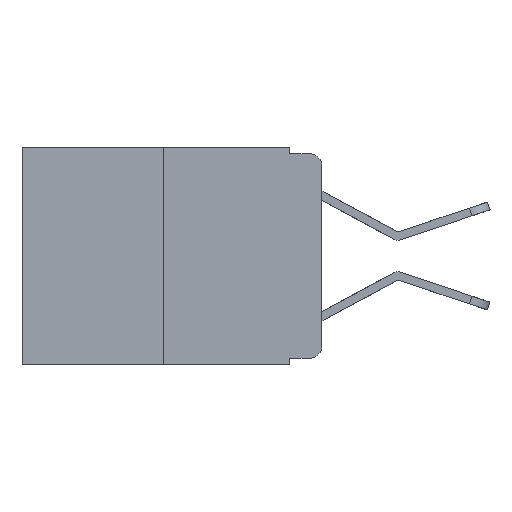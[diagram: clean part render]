
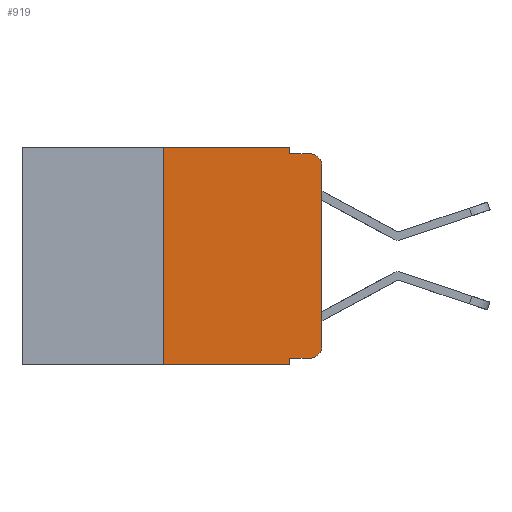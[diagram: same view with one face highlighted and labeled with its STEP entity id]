
A CAD part, left-side view. The second image highlights one B-rep face of the part: STEP entity #919.
In plain terms, the highlighted planar face has unit normal (-1, 0, 0).
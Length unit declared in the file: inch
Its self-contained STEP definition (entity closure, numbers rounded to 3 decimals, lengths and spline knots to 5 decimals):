
#36 = LINE ( 'NONE', #2235, #15586 ) ;
#129 = AXIS2_PLACEMENT_3D ( 'NONE', #6723, #17205, #8230 ) ;
#309 = LINE ( 'NONE', #2579, #7879 ) ;
#554 = ORIENTED_EDGE ( 'NONE', *, *, #718, .F. ) ;
#718 = EDGE_CURVE ( 'NONE', #16285, #2313, #2250, .T. ) ;
#919 = ADVANCED_FACE ( 'NONE', ( #9537 ), #12944, .F. ) ;
#1104 = DIRECTION ( 'NONE',  ( 1., 0., 0. ) ) ;
#1184 = EDGE_CURVE ( 'NONE', #2313, #10644, #309, .T. ) ;
#1621 = LINE ( 'NONE', #5008, #17148 ) ;
#2152 = EDGE_CURVE ( 'NONE', #19478, #2261, #36, .T. ) ;
#2235 = CARTESIAN_POINT ( 'NONE',  ( 0., 0.051, 0. ) ) ;
#2250 = LINE ( 'NONE', #16620, #9306 ) ;
#2261 = VERTEX_POINT ( 'NONE', #2502 ) ;
#2296 = DIRECTION ( 'NONE',  ( 0., 0., -1. ) ) ;
#2313 = VERTEX_POINT ( 'NONE', #13131 ) ;
#2376 = CARTESIAN_POINT ( 'NONE',  ( 0., 0.473, -0.343 ) ) ;
#2391 = EDGE_CURVE ( 'NONE', #10644, #11208, #12288, .T. ) ;
#2502 = CARTESIAN_POINT ( 'NONE',  ( 0., 0.051, -0.343 ) ) ;
#2579 = CARTESIAN_POINT ( 'NONE',  ( 0., 0.473, 0. ) ) ;
#2669 = DIRECTION ( 'NONE',  ( -1., 0., 0. ) ) ;
#3202 = VERTEX_POINT ( 'NONE', #13690 ) ;
#3598 = VECTOR ( 'NONE', #7620, 39.37008 ) ;
#3809 = VERTEX_POINT ( 'NONE', #4970 ) ;
#3857 = VECTOR ( 'NONE', #10298, 39.37008 ) ;
#3967 = CARTESIAN_POINT ( 'NONE',  ( 0., 0., -0.03 ) ) ;
#4226 = VERTEX_POINT ( 'NONE', #10428 ) ;
#4970 = CARTESIAN_POINT ( 'NONE',  ( 0., 0.02, -0.333 ) ) ;
#5008 = CARTESIAN_POINT ( 'NONE',  ( 0., 0., 0. ) ) ;
#5072 = ORIENTED_EDGE ( 'NONE', *, *, #16194, .F. ) ;
#5185 = EDGE_CURVE ( 'NONE', #4226, #17462, #1621, .T. ) ;
#5431 = DIRECTION ( 'NONE',  ( 0., -1., 0. ) ) ;
#5439 = CIRCLE ( 'NONE', #16748, 0.02 ) ;
#5445 = EDGE_CURVE ( 'NONE', #17462, #3202, #5439, .T. ) ;
#5690 = CARTESIAN_POINT ( 'NONE',  ( 0., 0.051, 0. ) ) ;
#6305 = CARTESIAN_POINT ( 'NONE',  ( 0., 0.25, -0.343 ) ) ;
#6453 = EDGE_CURVE ( 'NONE', #3809, #4226, #7027, .T. ) ;
#6723 = CARTESIAN_POINT ( 'NONE',  ( 0., 0.02, -0.313 ) ) ;
#7027 = CIRCLE ( 'NONE', #129, 0.02 ) ;
#7396 = CARTESIAN_POINT ( 'NONE',  ( 0., 0.051, -0.333 ) ) ;
#7620 = DIRECTION ( 'NONE',  ( 0., -1., 0. ) ) ;
#7879 = VECTOR ( 'NONE', #9435, 39.37008 ) ;
#8230 = DIRECTION ( 'NONE',  ( 0., 0., -1. ) ) ;
#9294 = ORIENTED_EDGE ( 'NONE', *, *, #2152, .F. ) ;
#9306 = VECTOR ( 'NONE', #10975, 39.37008 ) ;
#9435 = DIRECTION ( 'NONE',  ( 0., -1., 0. ) ) ;
#9537 = FACE_OUTER_BOUND ( 'NONE', #10480, .T. ) ;
#10207 = ORIENTED_EDGE ( 'NONE', *, *, #1184, .F. ) ;
#10298 = DIRECTION ( 'NONE',  ( 0., 0., -1. ) ) ;
#10428 = CARTESIAN_POINT ( 'NONE',  ( 0., 0., -0.313 ) ) ;
#10480 = EDGE_LOOP ( 'NONE', ( #12569, #10923, #5072, #11377, #10207, #554, #18935, #9294, #15152, #17035 ) ) ;
#10644 = VERTEX_POINT ( 'NONE', #5690 ) ;
#10831 = AXIS2_PLACEMENT_3D ( 'NONE', #12883, #1104, #15188 ) ;
#10850 = VECTOR ( 'NONE', #17911, 39.37008 ) ;
#10923 = ORIENTED_EDGE ( 'NONE', *, *, #5445, .T. ) ;
#10975 = DIRECTION ( 'NONE',  ( 0., 0., 1. ) ) ;
#11006 = DIRECTION ( 'NONE',  ( 0., 0., 1. ) ) ;
#11208 = VERTEX_POINT ( 'NONE', #17960 ) ;
#11298 = LINE ( 'NONE', #2376, #18355 ) ;
#11377 = ORIENTED_EDGE ( 'NONE', *, *, #2391, .F. ) ;
#11644 = CARTESIAN_POINT ( 'NONE',  ( 0., 0.02, -0.03 ) ) ;
#12288 = LINE ( 'NONE', #14771, #3857 ) ;
#12569 = ORIENTED_EDGE ( 'NONE', *, *, #5185, .T. ) ;
#12883 = CARTESIAN_POINT ( 'NONE',  ( 0., 0.473, 0. ) ) ;
#12944 = PLANE ( 'NONE',  #10831 ) ;
#13131 = CARTESIAN_POINT ( 'NONE',  ( 0., 0.25, 0. ) ) ;
#13175 = DIRECTION ( 'NONE',  ( 0., 0., -1. ) ) ;
#13690 = CARTESIAN_POINT ( 'NONE',  ( 0., 0.02, -0.01 ) ) ;
#14771 = CARTESIAN_POINT ( 'NONE',  ( 0., 0.051, 0. ) ) ;
#15152 = ORIENTED_EDGE ( 'NONE', *, *, #16474, .T. ) ;
#15188 = DIRECTION ( 'NONE',  ( 0., 0., -1. ) ) ;
#15349 = CARTESIAN_POINT ( 'NONE',  ( 0., 0.051, -0.333 ) ) ;
#15586 = VECTOR ( 'NONE', #2296, 39.37008 ) ;
#16194 = EDGE_CURVE ( 'NONE', #11208, #3202, #19111, .T. ) ;
#16285 = VERTEX_POINT ( 'NONE', #6305 ) ;
#16474 = EDGE_CURVE ( 'NONE', #19478, #3809, #18396, .T. ) ;
#16577 = CARTESIAN_POINT ( 'NONE',  ( 0., 0.051, -0.01 ) ) ;
#16620 = CARTESIAN_POINT ( 'NONE',  ( 0., 0.25, 0. ) ) ;
#16748 = AXIS2_PLACEMENT_3D ( 'NONE', #11644, #2669, #13175 ) ;
#17035 = ORIENTED_EDGE ( 'NONE', *, *, #6453, .T. ) ;
#17148 = VECTOR ( 'NONE', #11006, 39.37008 ) ;
#17205 = DIRECTION ( 'NONE',  ( -1., 0., 0. ) ) ;
#17431 = EDGE_CURVE ( 'NONE', #16285, #2261, #11298, .T. ) ;
#17462 = VERTEX_POINT ( 'NONE', #3967 ) ;
#17911 = DIRECTION ( 'NONE',  ( 0., -1., 0. ) ) ;
#17960 = CARTESIAN_POINT ( 'NONE',  ( 0., 0.051, -0.01 ) ) ;
#18355 = VECTOR ( 'NONE', #5431, 39.37008 ) ;
#18396 = LINE ( 'NONE', #7396, #10850 ) ;
#18935 = ORIENTED_EDGE ( 'NONE', *, *, #17431, .T. ) ;
#19111 = LINE ( 'NONE', #16577, #3598 ) ;
#19478 = VERTEX_POINT ( 'NONE', #15349 ) ;
